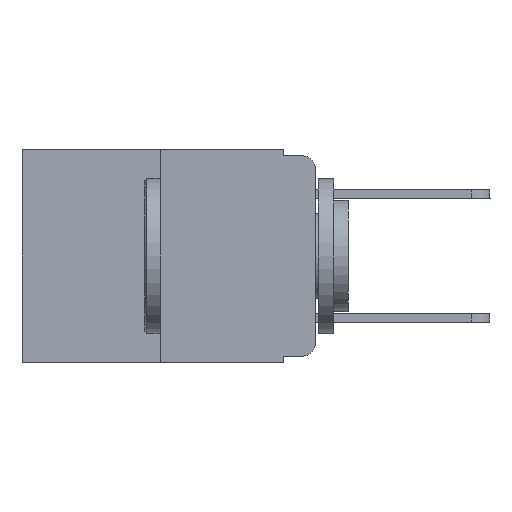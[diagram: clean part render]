
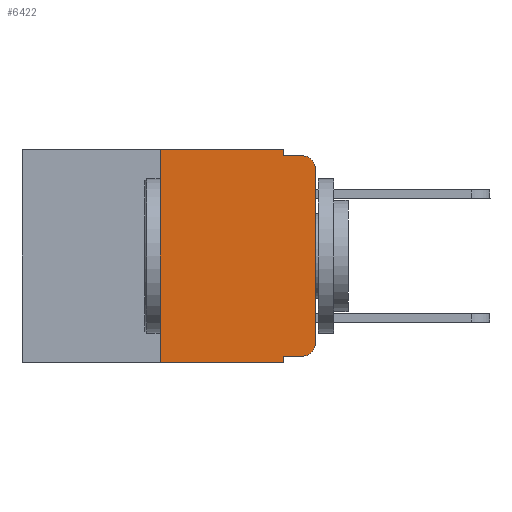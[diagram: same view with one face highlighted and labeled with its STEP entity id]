
A CAD part, left-side view. The second image highlights one B-rep face of the part: STEP entity #6422.
In plain terms, the highlighted planar face has unit normal (-1, 0, 0).
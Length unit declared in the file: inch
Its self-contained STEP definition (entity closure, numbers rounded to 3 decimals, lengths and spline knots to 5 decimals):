
#340 = CARTESIAN_POINT ( 'NONE',  ( 0., 0.02, -0.03 ) ) ;
#943 = DIRECTION ( 'NONE',  ( 1., 0., 0. ) ) ;
#970 = CARTESIAN_POINT ( 'NONE',  ( 0., 0.25, 0. ) ) ;
#1109 = EDGE_CURVE ( 'NONE', #4399, #4258, #16088, .T. ) ;
#1203 = VERTEX_POINT ( 'NONE', #1780 ) ;
#1220 = LINE ( 'NONE', #6928, #3431 ) ;
#1780 = CARTESIAN_POINT ( 'NONE',  ( 0., 0.051, -0.343 ) ) ;
#2121 = DIRECTION ( 'NONE',  ( 0., -1., 0. ) ) ;
#2566 = VECTOR ( 'NONE', #5312, 39.37008 ) ;
#2586 = ORIENTED_EDGE ( 'NONE', *, *, #10949, .F. ) ;
#2673 = VECTOR ( 'NONE', #11166, 39.37008 ) ;
#2936 = CARTESIAN_POINT ( 'NONE',  ( 0., 0.051, -0.333 ) ) ;
#2949 = VECTOR ( 'NONE', #8514, 39.37008 ) ;
#3009 = VECTOR ( 'NONE', #11560, 39.37008 ) ;
#3304 = CARTESIAN_POINT ( 'NONE',  ( 0., 0., -0.03 ) ) ;
#3423 = VERTEX_POINT ( 'NONE', #3304 ) ;
#3431 = VECTOR ( 'NONE', #12627, 39.37008 ) ;
#4057 = DIRECTION ( 'NONE',  ( 0., -1., 0. ) ) ;
#4191 = DIRECTION ( 'NONE',  ( 0., 0., -1. ) ) ;
#4258 = VERTEX_POINT ( 'NONE', #4659 ) ;
#4399 = VERTEX_POINT ( 'NONE', #10840 ) ;
#4500 = VERTEX_POINT ( 'NONE', #6434 ) ;
#4659 = CARTESIAN_POINT ( 'NONE',  ( 0., 0., -0.313 ) ) ;
#4702 = ORIENTED_EDGE ( 'NONE', *, *, #15313, .T. ) ;
#5297 = EDGE_LOOP ( 'NONE', ( #11808, #4702, #6746, #14191, #2586, #14293, #14006, #14620, #13500, #10102 ) ) ;
#5312 = DIRECTION ( 'NONE',  ( 0., -1., 0. ) ) ;
#5457 = LINE ( 'NONE', #11168, #15434 ) ;
#5893 = VECTOR ( 'NONE', #2121, 39.37008 ) ;
#6230 = LINE ( 'NONE', #11936, #5893 ) ;
#6422 = ADVANCED_FACE ( 'NONE', ( #6922 ), #8062, .F. ) ;
#6434 = CARTESIAN_POINT ( 'NONE',  ( 0., 0.25, -0.343 ) ) ;
#6484 = EDGE_CURVE ( 'NONE', #4258, #3423, #12612, .T. ) ;
#6715 = LINE ( 'NONE', #8316, #2566 ) ;
#6746 = ORIENTED_EDGE ( 'NONE', *, *, #8956, .F. ) ;
#6922 = FACE_OUTER_BOUND ( 'NONE', #5297, .T. ) ;
#6928 = CARTESIAN_POINT ( 'NONE',  ( 0., 0.051, -0.01 ) ) ;
#7163 = EDGE_CURVE ( 'NONE', #4500, #13565, #16772, .T. ) ;
#7306 = DIRECTION ( 'NONE',  ( -1., 0., 0. ) ) ;
#7444 = CIRCLE ( 'NONE', #13709, 0.02 ) ;
#8041 = AXIS2_PLACEMENT_3D ( 'NONE', #18318, #943, #18039 ) ;
#8062 = PLANE ( 'NONE',  #8041 ) ;
#8145 = EDGE_CURVE ( 'NONE', #10715, #4399, #6715, .T. ) ;
#8203 = EDGE_CURVE ( 'NONE', #10715, #1203, #18485, .T. ) ;
#8316 = CARTESIAN_POINT ( 'NONE',  ( 0., 0.051, -0.333 ) ) ;
#8490 = LINE ( 'NONE', #17160, #3009 ) ;
#8514 = DIRECTION ( 'NONE',  ( 0., 0., 1. ) ) ;
#8630 = CARTESIAN_POINT ( 'NONE',  ( 0., 0.02, -0.313 ) ) ;
#8702 = CARTESIAN_POINT ( 'NONE',  ( 0., 0., 0. ) ) ;
#8956 = EDGE_CURVE ( 'NONE', #9046, #11463, #1220, .T. ) ;
#9046 = VERTEX_POINT ( 'NONE', #18411 ) ;
#9717 = CARTESIAN_POINT ( 'NONE',  ( 0., 0.02, -0.01 ) ) ;
#10102 = ORIENTED_EDGE ( 'NONE', *, *, #1109, .T. ) ;
#10353 = DIRECTION ( 'NONE',  ( -1., 0., 0. ) ) ;
#10715 = VERTEX_POINT ( 'NONE', #2936 ) ;
#10840 = CARTESIAN_POINT ( 'NONE',  ( 0., 0.02, -0.333 ) ) ;
#10949 = EDGE_CURVE ( 'NONE', #13565, #16403, #5457, .T. ) ;
#11166 = DIRECTION ( 'NONE',  ( 0., 0., 1. ) ) ;
#11168 = CARTESIAN_POINT ( 'NONE',  ( 0., 0.473, 0. ) ) ;
#11463 = VERTEX_POINT ( 'NONE', #9717 ) ;
#11560 = DIRECTION ( 'NONE',  ( 0., 0., -1. ) ) ;
#11646 = EDGE_CURVE ( 'NONE', #4500, #1203, #6230, .T. ) ;
#11808 = ORIENTED_EDGE ( 'NONE', *, *, #6484, .T. ) ;
#11936 = CARTESIAN_POINT ( 'NONE',  ( 0., 0.473, -0.343 ) ) ;
#12339 = CARTESIAN_POINT ( 'NONE',  ( 0., 0.051, 0. ) ) ;
#12612 = LINE ( 'NONE', #8702, #2949 ) ;
#12627 = DIRECTION ( 'NONE',  ( 0., -1., 0. ) ) ;
#13005 = DIRECTION ( 'NONE',  ( 0., 0., -1. ) ) ;
#13500 = ORIENTED_EDGE ( 'NONE', *, *, #8145, .T. ) ;
#13565 = VERTEX_POINT ( 'NONE', #13586 ) ;
#13586 = CARTESIAN_POINT ( 'NONE',  ( 0., 0.25, 0. ) ) ;
#13709 = AXIS2_PLACEMENT_3D ( 'NONE', #340, #10353, #16142 ) ;
#14006 = ORIENTED_EDGE ( 'NONE', *, *, #11646, .T. ) ;
#14191 = ORIENTED_EDGE ( 'NONE', *, *, #18108, .F. ) ;
#14293 = ORIENTED_EDGE ( 'NONE', *, *, #7163, .F. ) ;
#14446 = CARTESIAN_POINT ( 'NONE',  ( 0., 0.051, 0. ) ) ;
#14620 = ORIENTED_EDGE ( 'NONE', *, *, #8203, .F. ) ;
#15313 = EDGE_CURVE ( 'NONE', #3423, #11463, #7444, .T. ) ;
#15434 = VECTOR ( 'NONE', #4057, 39.37008 ) ;
#16088 = CIRCLE ( 'NONE', #18482, 0.02 ) ;
#16142 = DIRECTION ( 'NONE',  ( 0., 0., -1. ) ) ;
#16403 = VERTEX_POINT ( 'NONE', #12339 ) ;
#16772 = LINE ( 'NONE', #970, #2673 ) ;
#16838 = VECTOR ( 'NONE', #4191, 39.37008 ) ;
#17160 = CARTESIAN_POINT ( 'NONE',  ( 0., 0.051, 0. ) ) ;
#18039 = DIRECTION ( 'NONE',  ( 0., 0., -1. ) ) ;
#18108 = EDGE_CURVE ( 'NONE', #16403, #9046, #8490, .T. ) ;
#18318 = CARTESIAN_POINT ( 'NONE',  ( 0., 0.473, 0. ) ) ;
#18411 = CARTESIAN_POINT ( 'NONE',  ( 0., 0.051, -0.01 ) ) ;
#18482 = AXIS2_PLACEMENT_3D ( 'NONE', #8630, #7306, #13005 ) ;
#18485 = LINE ( 'NONE', #14446, #16838 ) ;
